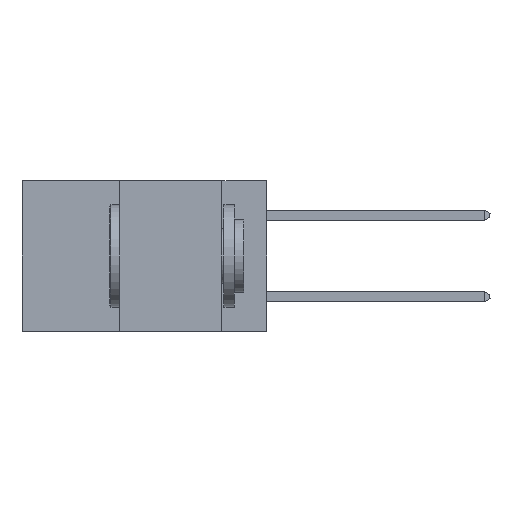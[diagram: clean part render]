
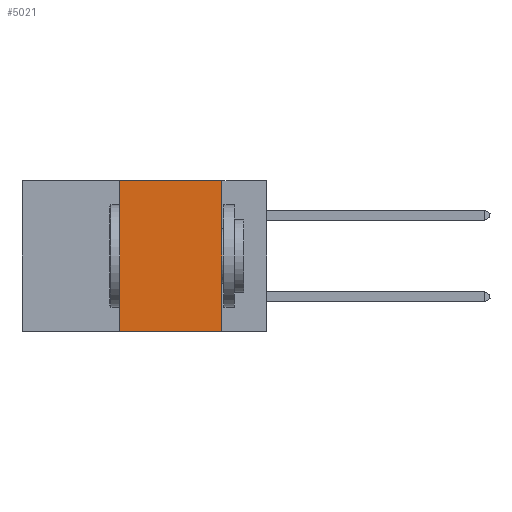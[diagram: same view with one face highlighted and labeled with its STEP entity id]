
A CAD part, left-side view. The second image highlights one B-rep face of the part: STEP entity #5021.
In plain terms, the highlighted planar face has unit normal (-1, 0, 0).
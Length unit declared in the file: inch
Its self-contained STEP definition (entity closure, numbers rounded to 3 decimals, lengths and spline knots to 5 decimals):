
#102 = ORIENTED_EDGE ( 'NONE', *, *, #15919, .F. ) ;
#625 = CARTESIAN_POINT ( 'NONE',  ( 0., 0.36, 0. ) ) ;
#1260 = DIRECTION ( 'NONE',  ( 0., 0., -1. ) ) ;
#2869 = LINE ( 'NONE', #17624, #7339 ) ;
#2915 = LINE ( 'NONE', #625, #7972 ) ;
#3380 = FACE_OUTER_BOUND ( 'NONE', #23491, .T. ) ;
#3564 = DIRECTION ( 'NONE',  ( 0., -1., 0. ) ) ;
#4536 = VERTEX_POINT ( 'NONE', #17638 ) ;
#4560 = CARTESIAN_POINT ( 'NONE',  ( 0., 0.36, -0.37 ) ) ;
#5021 = ADVANCED_FACE ( 'NONE', ( #3380 ), #23436, .F. ) ;
#5522 = VERTEX_POINT ( 'NONE', #4560 ) ;
#6185 = EDGE_CURVE ( 'NONE', #5522, #4536, #2915, .T. ) ;
#7339 = VECTOR ( 'NONE', #10234, 39.37008 ) ;
#7721 = ORIENTED_EDGE ( 'NONE', *, *, #6185, .F. ) ;
#7972 = VECTOR ( 'NONE', #13809, 39.37008 ) ;
#8735 = LINE ( 'NONE', #12945, #23332 ) ;
#8812 = CARTESIAN_POINT ( 'NONE',  ( 0., 0.6, 0. ) ) ;
#10234 = DIRECTION ( 'NONE',  ( 0., -1., 0. ) ) ;
#12808 = DIRECTION ( 'NONE',  ( 0., 0., -1. ) ) ;
#12945 = CARTESIAN_POINT ( 'NONE',  ( 0., 0.6, 0. ) ) ;
#12950 = EDGE_CURVE ( 'NONE', #16557, #21315, #23162, .T. ) ;
#13532 = VECTOR ( 'NONE', #12808, 39.37008 ) ;
#13809 = DIRECTION ( 'NONE',  ( 0., 0., 1. ) ) ;
#14340 = DIRECTION ( 'NONE',  ( 1., 0., 0. ) ) ;
#14559 = ORIENTED_EDGE ( 'NONE', *, *, #12950, .F. ) ;
#14572 = CARTESIAN_POINT ( 'NONE',  ( 0., 0.11, 0. ) ) ;
#14609 = AXIS2_PLACEMENT_3D ( 'NONE', #8812, #14340, #1260 ) ;
#15919 = EDGE_CURVE ( 'NONE', #4536, #16557, #8735, .T. ) ;
#16557 = VERTEX_POINT ( 'NONE', #22349 ) ;
#17624 = CARTESIAN_POINT ( 'NONE',  ( 0., 0.6, -0.37 ) ) ;
#17638 = CARTESIAN_POINT ( 'NONE',  ( 0., 0.36, 0. ) ) ;
#21315 = VERTEX_POINT ( 'NONE', #22182 ) ;
#22182 = CARTESIAN_POINT ( 'NONE',  ( 0., 0.11, -0.37 ) ) ;
#22337 = ORIENTED_EDGE ( 'NONE', *, *, #22946, .T. ) ;
#22349 = CARTESIAN_POINT ( 'NONE',  ( 0., 0.11, 0. ) ) ;
#22946 = EDGE_CURVE ( 'NONE', #5522, #21315, #2869, .T. ) ;
#23162 = LINE ( 'NONE', #14572, #13532 ) ;
#23332 = VECTOR ( 'NONE', #3564, 39.37008 ) ;
#23436 = PLANE ( 'NONE',  #14609 ) ;
#23491 = EDGE_LOOP ( 'NONE', ( #14559, #102, #7721, #22337 ) ) ;
